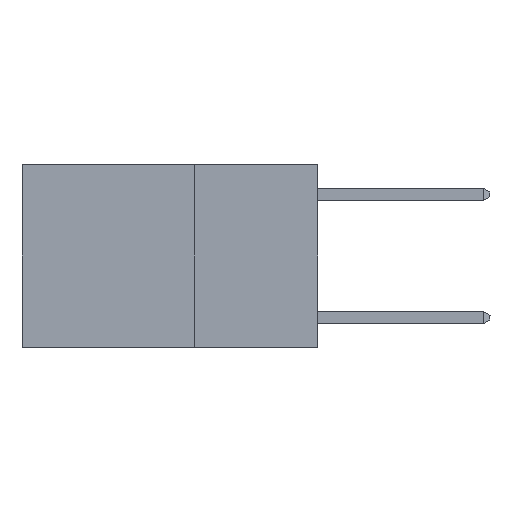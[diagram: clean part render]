
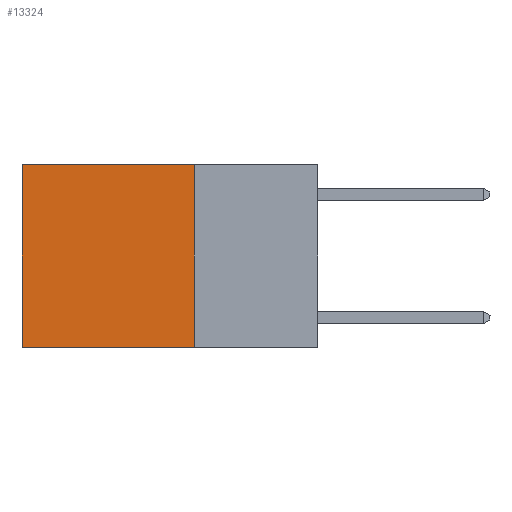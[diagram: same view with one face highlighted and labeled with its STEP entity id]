
A CAD part, left-side view. The second image highlights one B-rep face of the part: STEP entity #13324.
In plain terms, the highlighted planar face has unit normal (-1, 0, 0).
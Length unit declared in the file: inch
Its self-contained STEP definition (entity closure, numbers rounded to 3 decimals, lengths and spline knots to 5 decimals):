
#540 = EDGE_CURVE ( 'NONE', #13885, #11769, #11722, .T. ) ;
#970 = CARTESIAN_POINT ( 'NONE',  ( 0.2625, 0.6, 0. ) ) ;
#1433 = VECTOR ( 'NONE', #15316, 39.37008 ) ;
#1449 = CARTESIAN_POINT ( 'NONE',  ( 0.2625, 0.25, 0. ) ) ;
#1622 = CARTESIAN_POINT ( 'NONE',  ( 0.2625, 0.25, 0. ) ) ;
#2848 = VERTEX_POINT ( 'NONE', #19153 ) ;
#3433 = EDGE_CURVE ( 'NONE', #2848, #13885, #8083, .T. ) ;
#4063 = LINE ( 'NONE', #10770, #10711 ) ;
#4340 = FACE_OUTER_BOUND ( 'NONE', #10657, .T. ) ;
#5590 = VECTOR ( 'NONE', #18374, 39.37008 ) ;
#5915 = DIRECTION ( 'NONE',  ( 1., 0., 0. ) ) ;
#7860 = DIRECTION ( 'NONE',  ( 0., 0., -1. ) ) ;
#8078 = VERTEX_POINT ( 'NONE', #8237 ) ;
#8083 = LINE ( 'NONE', #19672, #1433 ) ;
#8237 = CARTESIAN_POINT ( 'NONE',  ( 0.2625, 0.25, -0.37 ) ) ;
#8296 = ORIENTED_EDGE ( 'NONE', *, *, #17502, .F. ) ;
#9469 = ORIENTED_EDGE ( 'NONE', *, *, #540, .T. ) ;
#10657 = EDGE_LOOP ( 'NONE', ( #9469, #8296, #19499, #11100 ) ) ;
#10711 = VECTOR ( 'NONE', #12467, 39.37008 ) ;
#10770 = CARTESIAN_POINT ( 'NONE',  ( 0.2625, 0.25, -0.37 ) ) ;
#11100 = ORIENTED_EDGE ( 'NONE', *, *, #3433, .T. ) ;
#11722 = LINE ( 'NONE', #16692, #5590 ) ;
#11769 = VERTEX_POINT ( 'NONE', #18540 ) ;
#12467 = DIRECTION ( 'NONE',  ( 0., 1., 0. ) ) ;
#12776 = VECTOR ( 'NONE', #7860, 39.37008 ) ;
#13038 = LINE ( 'NONE', #1622, #12776 ) ;
#13324 = ADVANCED_FACE ( 'NONE', ( #4340 ), #16505, .F. ) ;
#13885 = VERTEX_POINT ( 'NONE', #970 ) ;
#15316 = DIRECTION ( 'NONE',  ( 0., 1., 0. ) ) ;
#16505 = PLANE ( 'NONE',  #17484 ) ;
#16571 = DIRECTION ( 'NONE',  ( 0., 0., -1. ) ) ;
#16692 = CARTESIAN_POINT ( 'NONE',  ( 0.2625, 0.6, 0. ) ) ;
#17397 = EDGE_CURVE ( 'NONE', #2848, #8078, #13038, .T. ) ;
#17484 = AXIS2_PLACEMENT_3D ( 'NONE', #1449, #5915, #16571 ) ;
#17502 = EDGE_CURVE ( 'NONE', #8078, #11769, #4063, .T. ) ;
#18374 = DIRECTION ( 'NONE',  ( 0., 0., -1. ) ) ;
#18540 = CARTESIAN_POINT ( 'NONE',  ( 0.2625, 0.6, -0.37 ) ) ;
#19153 = CARTESIAN_POINT ( 'NONE',  ( 0.2625, 0.25, 0. ) ) ;
#19499 = ORIENTED_EDGE ( 'NONE', *, *, #17397, .F. ) ;
#19672 = CARTESIAN_POINT ( 'NONE',  ( 0.2625, 0.25, 0. ) ) ;
